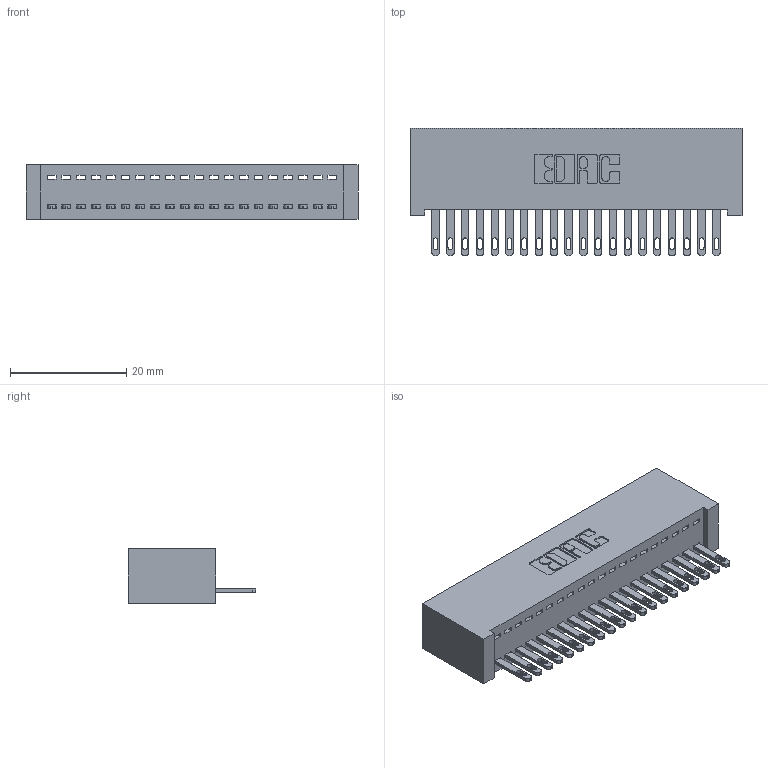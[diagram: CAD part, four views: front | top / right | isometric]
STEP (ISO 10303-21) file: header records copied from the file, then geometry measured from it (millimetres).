
FILE_DESCRIPTION (( 'STEP AP203' ), '1' );
FILE_NAME ('892-020-500-101.STEP', '2020-09-21T13:51:37', ( '' ), ( '' ), 'SwSTEP 2.0', 'SolidWorks 2020', '' );
FILE_SCHEMA (( 'CONFIG_CONTROL_DESIGN' ));
Length unit declared in the file: inch
Products named in the file (3): 842 Part_Lugless; 345-292-001_345-293-100; 892-020-500-101
Assembly tree (21 placements, depth 2):
  892-020-500-101
    842 Part_Lugless
    345-292-001_345-293-100  x20
Bounding box: 57.05 x 21.85 x 9.4 mm (x, y, z)
Volume: 5342.3 mm3; surface area: 7796.9 mm2
Topology: 21 solids, 21 shells, 1182 faces, 3635 edges, 2422 vertices
Faces by surface type: plane 782, cylinder 400
Entity records: 14593 total; most frequent: CARTESIAN_POINT 2526, ORIENTED_EDGE 2482, DIRECTION 2169, EDGE_CURVE 1241, LINE 1117, VECTOR 1117, VERTEX_POINT 826, AXIS2_PLACEMENT_3D 526
